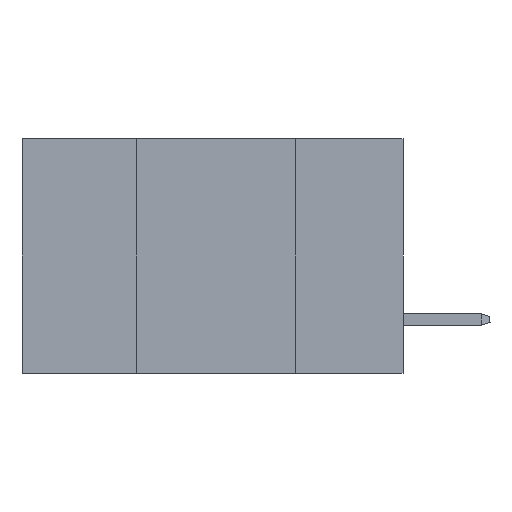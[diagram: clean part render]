
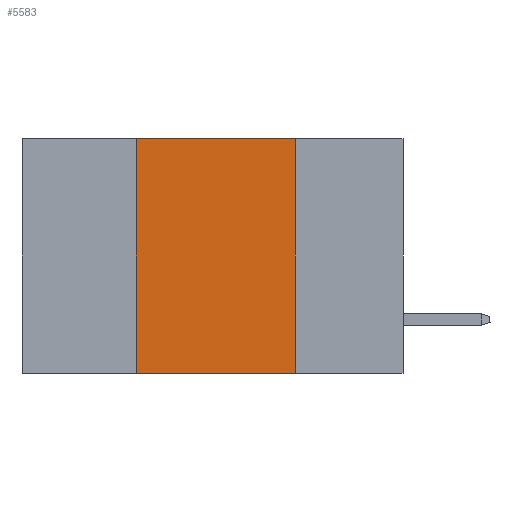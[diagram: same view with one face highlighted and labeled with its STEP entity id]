
A CAD part, left-side view. The second image highlights one B-rep face of the part: STEP entity #5583.
In plain terms, the highlighted planar face has unit normal (-1, 0, 0).
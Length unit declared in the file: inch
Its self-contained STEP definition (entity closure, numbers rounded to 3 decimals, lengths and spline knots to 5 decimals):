
#631 = EDGE_CURVE ( 'NONE', #40516, #46127, #13819, .T. ) ;
#1890 = ORIENTED_EDGE ( 'NONE', *, *, #11763, .F. ) ;
#3178 = CARTESIAN_POINT ( 'NONE',  ( 0., 0.6, 0. ) ) ;
#3347 = VECTOR ( 'NONE', #24961, 39.37008 ) ;
#4102 = FACE_OUTER_BOUND ( 'NONE', #42238, .T. ) ;
#5583 = ADVANCED_FACE ( 'NONE', ( #4102 ), #14057, .F. ) ;
#6056 = AXIS2_PLACEMENT_3D ( 'NONE', #32906, #11438, #35752 ) ;
#6404 = EDGE_CURVE ( 'NONE', #37175, #29607, #21953, .T. ) ;
#6662 = EDGE_CURVE ( 'NONE', #46127, #29607, #46441, .T. ) ;
#10511 = VECTOR ( 'NONE', #18971, 39.37008 ) ;
#11438 = DIRECTION ( 'NONE',  ( 1., 0., 0. ) ) ;
#11763 = EDGE_CURVE ( 'NONE', #37175, #40516, #44680, .T. ) ;
#13150 = ORIENTED_EDGE ( 'NONE', *, *, #631, .F. ) ;
#13496 = ORIENTED_EDGE ( 'NONE', *, *, #6662, .F. ) ;
#13819 = LINE ( 'NONE', #3178, #37644 ) ;
#14057 = PLANE ( 'NONE',  #6056 ) ;
#18971 = DIRECTION ( 'NONE',  ( 0., 0., 1. ) ) ;
#21395 = VECTOR ( 'NONE', #22647, 39.37008 ) ;
#21953 = LINE ( 'NONE', #40809, #21395 ) ;
#22607 = CARTESIAN_POINT ( 'NONE',  ( 0., 0.42, 0. ) ) ;
#22647 = DIRECTION ( 'NONE',  ( 0., -1., 0. ) ) ;
#24961 = DIRECTION ( 'NONE',  ( 0., 0., -1. ) ) ;
#29607 = VERTEX_POINT ( 'NONE', #43289 ) ;
#32870 = CARTESIAN_POINT ( 'NONE',  ( 0., 0.17, 0. ) ) ;
#32906 = CARTESIAN_POINT ( 'NONE',  ( 0., 0.6, 0. ) ) ;
#35752 = DIRECTION ( 'NONE',  ( 0., 0., -1. ) ) ;
#37175 = VERTEX_POINT ( 'NONE', #40104 ) ;
#37644 = VECTOR ( 'NONE', #38143, 39.37008 ) ;
#38143 = DIRECTION ( 'NONE',  ( 0., -1., 0. ) ) ;
#39980 = ORIENTED_EDGE ( 'NONE', *, *, #6404, .T. ) ;
#40104 = CARTESIAN_POINT ( 'NONE',  ( 0., 0.42, -0.37 ) ) ;
#40516 = VERTEX_POINT ( 'NONE', #22607 ) ;
#40809 = CARTESIAN_POINT ( 'NONE',  ( 0., 0.6, -0.37 ) ) ;
#42238 = EDGE_LOOP ( 'NONE', ( #13496, #13150, #1890, #39980 ) ) ;
#43289 = CARTESIAN_POINT ( 'NONE',  ( 0., 0.17, -0.37 ) ) ;
#44680 = LINE ( 'NONE', #44916, #10511 ) ;
#44916 = CARTESIAN_POINT ( 'NONE',  ( 0., 0.42, 0. ) ) ;
#46127 = VERTEX_POINT ( 'NONE', #32870 ) ;
#46209 = CARTESIAN_POINT ( 'NONE',  ( 0., 0.17, 0. ) ) ;
#46441 = LINE ( 'NONE', #46209, #3347 ) ;
